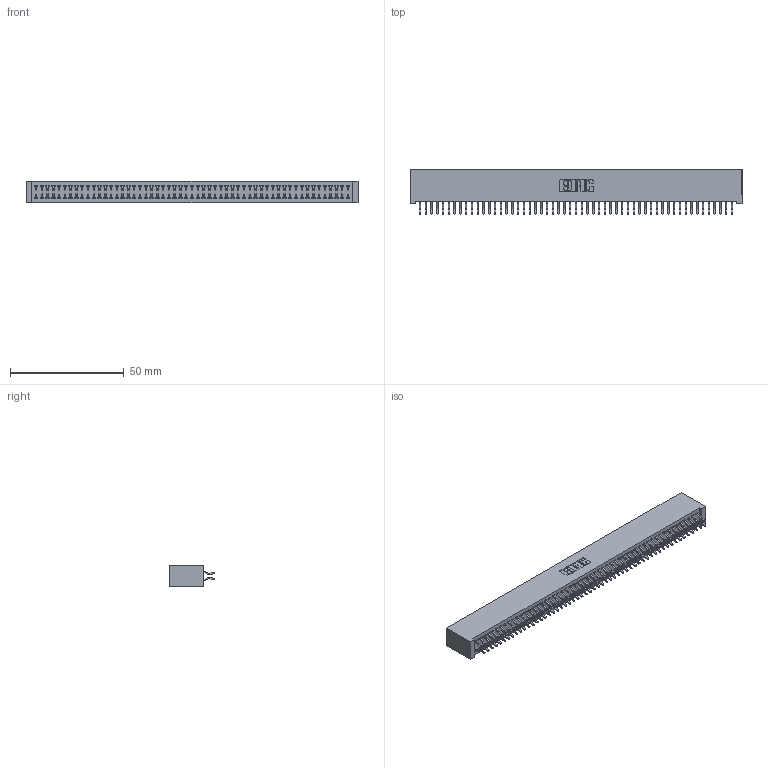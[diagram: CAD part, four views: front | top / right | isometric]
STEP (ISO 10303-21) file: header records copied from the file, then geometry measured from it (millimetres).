
FILE_DESCRIPTION (( 'STEP AP203' ), '1' );
FILE_NAME ('342-110-556-201.STEP', '2019-10-04T20:31:22', ( '' ), ( '' ), 'SwSTEP 2.0', 'SolidWorks 2016', '' );
FILE_SCHEMA (( 'CONFIG_CONTROL_DESIGN' ));
Length unit declared in the file: inch
Products named in the file (3): 342-110-556-201; 342 Part_Lugless; 345-292-001_556 Tail
Assembly tree (111 placements, depth 2):
  342-110-556-201
    342 Part_Lugless
    345-292-001_556 Tail  x110
Bounding box: 145.95 x 19.58 x 9.4 mm (x, y, z)
Volume: 13611.7 mm3; surface area: 22816.3 mm2
Topology: 111 solids, 111 shells, 6482 faces, 19305 edges, 12722 vertices
Faces by surface type: plane 4462, cylinder 2020
Entity records: 33513 total; most frequent: CARTESIAN_POINT 5550, ORIENTED_EDGE 5474, DIRECTION 4701, EDGE_CURVE 2737, VECTOR 2609, LINE 2609, VERTEX_POINT 1822, AXIS2_PLACEMENT_3D 1046
